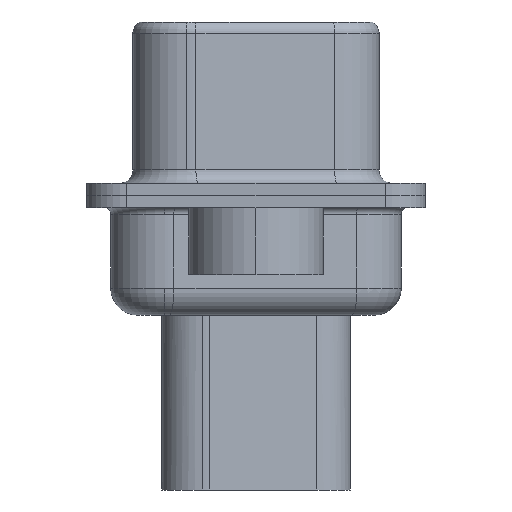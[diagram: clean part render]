
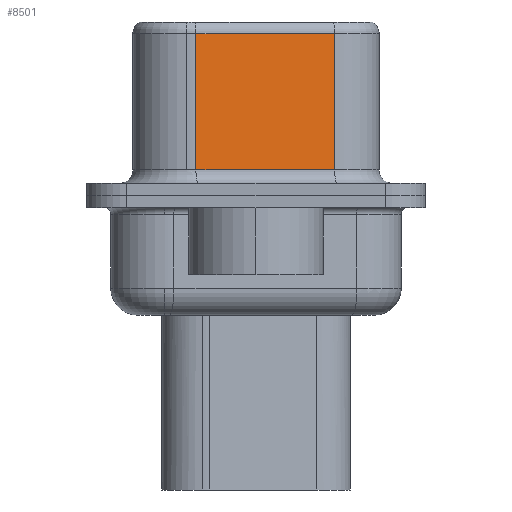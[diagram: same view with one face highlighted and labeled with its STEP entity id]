
A CAD part, left-side view. The second image highlights one B-rep face of the part: STEP entity #8501.
In plain terms, the highlighted planar face has unit normal (-0.985, -0.174, 0).
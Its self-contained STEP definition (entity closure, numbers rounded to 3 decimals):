
#28 = AXIS2_PLACEMENT_3D ( 'NONE', #5126, #451, #564 ) ;
#451 = DIRECTION ( 'NONE',  ( 0.985, 0.174, 0. ) ) ;
#527 = VERTEX_POINT ( 'NONE', #5525 ) ;
#564 = DIRECTION ( 'NONE',  ( -0.174, 0.985, 0. ) ) ;
#571 = EDGE_CURVE ( 'NONE', #2007, #591, #11956, .T. ) ;
#591 = VERTEX_POINT ( 'NONE', #1776 ) ;
#624 = LINE ( 'NONE', #7939, #11193 ) ;
#1698 = VECTOR ( 'NONE', #4607, 1000. ) ;
#1776 = CARTESIAN_POINT ( 'NONE',  ( 3.665, 2.233, 0.95 ) ) ;
#2007 = VERTEX_POINT ( 'NONE', #9571 ) ;
#2048 = CARTESIAN_POINT ( 'NONE',  ( 4.575, -2.927, 0.95 ) ) ;
#2360 = FACE_OUTER_BOUND ( 'NONE', #2578, .T. ) ;
#2446 = ORIENTED_EDGE ( 'NONE', *, *, #8438, .F. ) ;
#2578 = EDGE_LOOP ( 'NONE', ( #2446, #3623, #10680, #3484 ) ) ;
#3484 = ORIENTED_EDGE ( 'NONE', *, *, #10391, .T. ) ;
#3599 = DIRECTION ( 'NONE',  ( -0.174, 0.985, 0. ) ) ;
#3623 = ORIENTED_EDGE ( 'NONE', *, *, #9650, .T. ) ;
#4377 = VECTOR ( 'NONE', #3599, 1000. ) ;
#4607 = DIRECTION ( 'NONE',  ( 0., 0., -1. ) ) ;
#5126 = CARTESIAN_POINT ( 'NONE',  ( 4.575, -2.927, 6.52 ) ) ;
#5498 = CARTESIAN_POINT ( 'NONE',  ( 4.575, -2.927, 6.02 ) ) ;
#5525 = CARTESIAN_POINT ( 'NONE',  ( 4.575, -2.927, 0.95 ) ) ;
#6102 = PLANE ( 'NONE',  #28 ) ;
#7627 = VECTOR ( 'NONE', #10622, 1000. ) ;
#7820 = DIRECTION ( 'NONE',  ( 0., 0., -1. ) ) ;
#7939 = CARTESIAN_POINT ( 'NONE',  ( 4.575, -2.927, 6.52 ) ) ;
#8195 = VERTEX_POINT ( 'NONE', #9217 ) ;
#8250 = LINE ( 'NONE', #5498, #4377 ) ;
#8438 = EDGE_CURVE ( 'NONE', #8195, #527, #624, .T. ) ;
#8501 = ADVANCED_FACE ( 'NONE', ( #2360 ), #6102, .F. ) ;
#9217 = CARTESIAN_POINT ( 'NONE',  ( 4.575, -2.927, 6.02 ) ) ;
#9370 = CARTESIAN_POINT ( 'NONE',  ( 3.665, 2.233, 6.52 ) ) ;
#9571 = CARTESIAN_POINT ( 'NONE',  ( 3.665, 2.233, 6.02 ) ) ;
#9650 = EDGE_CURVE ( 'NONE', #8195, #2007, #8250, .T. ) ;
#10391 = EDGE_CURVE ( 'NONE', #591, #527, #11358, .T. ) ;
#10622 = DIRECTION ( 'NONE',  ( 0.174, -0.985, 0. ) ) ;
#10680 = ORIENTED_EDGE ( 'NONE', *, *, #571, .T. ) ;
#11193 = VECTOR ( 'NONE', #7820, 1000. ) ;
#11358 = LINE ( 'NONE', #2048, #7627 ) ;
#11956 = LINE ( 'NONE', #9370, #1698 ) ;
